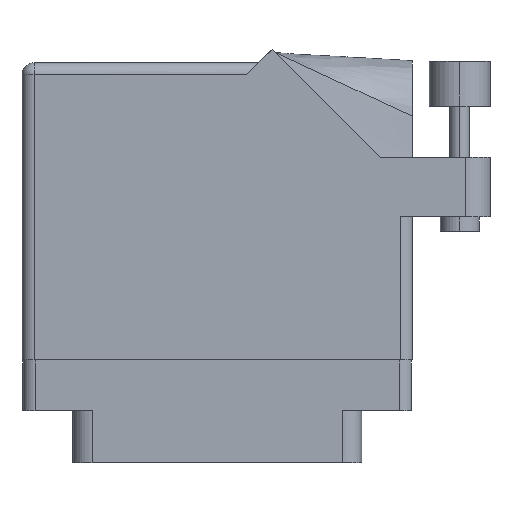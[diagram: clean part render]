
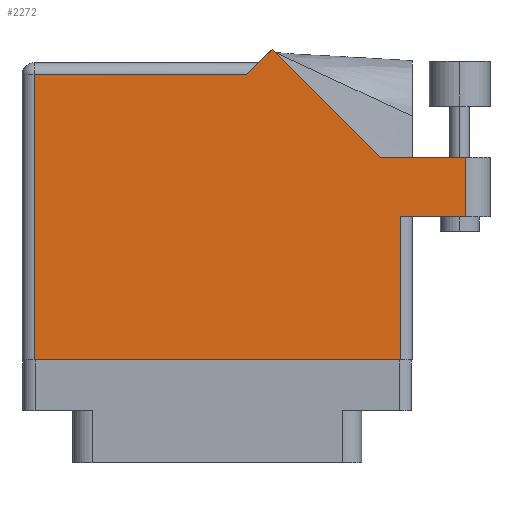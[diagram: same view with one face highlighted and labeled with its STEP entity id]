
A CAD part, front view. The second image highlights one B-rep face of the part: STEP entity #2272.
In plain terms, the highlighted face is planar.
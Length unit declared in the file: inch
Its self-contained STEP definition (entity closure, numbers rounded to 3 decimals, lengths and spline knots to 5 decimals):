
#702 = LINE ( 'NONE', #13015, #9710 ) ;
#1072 = DIRECTION ( 'NONE',  ( -0.707, 0.707, 0. ) ) ;
#1419 = CARTESIAN_POINT ( 'NONE',  ( 1.28771, 1.60071, 0. ) ) ;
#2039 = CARTESIAN_POINT ( 'NONE',  ( 1.948, 0.737, 0. ) ) ;
#2272 = ADVANCED_FACE ( 'NONE', ( #17366 ), #23611, .F. ) ;
#2548 = DIRECTION ( 'NONE',  ( 0., 0., -1. ) ) ;
#2586 = AXIS2_PLACEMENT_3D ( 'NONE', #30344, #2548, #4826 ) ;
#2947 = ORIENTED_EDGE ( 'NONE', *, *, #27175, .T. ) ;
#3048 = VECTOR ( 'NONE', #11093, 39.37008 ) ;
#3707 = CARTESIAN_POINT ( 'NONE',  ( 1.948, 0.737, 0. ) ) ;
#3743 = CARTESIAN_POINT ( 'NONE',  ( 2.285, 0.737, 0. ) ) ;
#4639 = DIRECTION ( 'NONE',  ( 1., 0., 0. ) ) ;
#4816 = CARTESIAN_POINT ( 'NONE',  ( 0.062, 1.468, 0. ) ) ;
#4826 = DIRECTION ( 'NONE',  ( -1., 0., 0. ) ) ;
#6056 = VERTEX_POINT ( 'NONE', #13619 ) ;
#6892 = DIRECTION ( 'NONE',  ( 1., 0., 0. ) ) ;
#6984 = VERTEX_POINT ( 'NONE', #25923 ) ;
#8253 = DIRECTION ( 'NONE',  ( -0.707, -0.707, 0. ) ) ;
#8354 = CARTESIAN_POINT ( 'NONE',  ( 1.84442, 1.044, 0. ) ) ;
#8413 = LINE ( 'NONE', #28722, #28688 ) ;
#9272 = VECTOR ( 'NONE', #6892, 39.37008 ) ;
#9411 = LINE ( 'NONE', #15979, #3048 ) ;
#9710 = VECTOR ( 'NONE', #1072, 39.37008 ) ;
#10117 = CARTESIAN_POINT ( 'NONE',  ( 2.285, 1.044, 0. ) ) ;
#10292 = VERTEX_POINT ( 'NONE', #4816 ) ;
#10432 = DIRECTION ( 'NONE',  ( 0., 1., 0. ) ) ;
#11093 = DIRECTION ( 'NONE',  ( 0., -1., 0. ) ) ;
#11745 = CARTESIAN_POINT ( 'NONE',  ( 2.01, 0.737, 0. ) ) ;
#12101 = ORIENTED_EDGE ( 'NONE', *, *, #15664, .T. ) ;
#13015 = CARTESIAN_POINT ( 'NONE',  ( 1.84442, 1.044, 0. ) ) ;
#13281 = CARTESIAN_POINT ( 'NONE',  ( 2.41, 1.044, 0. ) ) ;
#13391 = DIRECTION ( 'NONE',  ( -1., 0., 0. ) ) ;
#13619 = CARTESIAN_POINT ( 'NONE',  ( 0.062, 0., 0. ) ) ;
#13822 = VERTEX_POINT ( 'NONE', #1419 ) ;
#14353 = VECTOR ( 'NONE', #13391, 39.37008 ) ;
#15296 = VERTEX_POINT ( 'NONE', #20180 ) ;
#15664 = EDGE_CURVE ( 'NONE', #15296, #10292, #8413, .T. ) ;
#15979 = CARTESIAN_POINT ( 'NONE',  ( 0.062, 0., 0. ) ) ;
#16388 = LINE ( 'NONE', #2039, #27612 ) ;
#17276 = EDGE_CURVE ( 'NONE', #6984, #21477, #27123, .T. ) ;
#17366 = FACE_OUTER_BOUND ( 'NONE', #18644, .T. ) ;
#17962 = LINE ( 'NONE', #24942, #30354 ) ;
#18219 = VERTEX_POINT ( 'NONE', #3707 ) ;
#18430 = ORIENTED_EDGE ( 'NONE', *, *, #26678, .T. ) ;
#18644 = EDGE_LOOP ( 'NONE', ( #23502, #18430, #31048, #25879, #19253, #12101, #25400, #2947, #30390 ) ) ;
#19153 = EDGE_CURVE ( 'NONE', #10292, #6056, #9411, .T. ) ;
#19253 = ORIENTED_EDGE ( 'NONE', *, *, #28691, .T. ) ;
#19453 = CARTESIAN_POINT ( 'NONE',  ( 1.948, 0., 0. ) ) ;
#20180 = CARTESIAN_POINT ( 'NONE',  ( 1.155, 1.468, 0. ) ) ;
#21407 = DIRECTION ( 'NONE',  ( 0., 1., 0. ) ) ;
#21477 = VERTEX_POINT ( 'NONE', #8354 ) ;
#21483 = DIRECTION ( 'NONE',  ( -1., 0., 0. ) ) ;
#22442 = VECTOR ( 'NONE', #10432, 39.37008 ) ;
#23502 = ORIENTED_EDGE ( 'NONE', *, *, #24246, .T. ) ;
#23611 = PLANE ( 'NONE',  #2586 ) ;
#24246 = EDGE_CURVE ( 'NONE', #18219, #25685, #29378, .T. ) ;
#24713 = LINE ( 'NONE', #10117, #22442 ) ;
#24942 = CARTESIAN_POINT ( 'NONE',  ( 1.217, 1.53, 0. ) ) ;
#25400 = ORIENTED_EDGE ( 'NONE', *, *, #19153, .T. ) ;
#25685 = VERTEX_POINT ( 'NONE', #3743 ) ;
#25879 = ORIENTED_EDGE ( 'NONE', *, *, #26257, .T. ) ;
#25923 = CARTESIAN_POINT ( 'NONE',  ( 2.285, 1.044, 0. ) ) ;
#25981 = CARTESIAN_POINT ( 'NONE',  ( 0., 0., 0. ) ) ;
#26257 = EDGE_CURVE ( 'NONE', #21477, #13822, #702, .T. ) ;
#26678 = EDGE_CURVE ( 'NONE', #25685, #6984, #24713, .T. ) ;
#27123 = LINE ( 'NONE', #13281, #14353 ) ;
#27175 = EDGE_CURVE ( 'NONE', #6056, #29616, #28429, .T. ) ;
#27612 = VECTOR ( 'NONE', #21407, 39.37008 ) ;
#27784 = EDGE_CURVE ( 'NONE', #29616, #18219, #16388, .T. ) ;
#27885 = VECTOR ( 'NONE', #4639, 39.37008 ) ;
#28429 = LINE ( 'NONE', #25981, #9272 ) ;
#28688 = VECTOR ( 'NONE', #21483, 39.37008 ) ;
#28691 = EDGE_CURVE ( 'NONE', #13822, #15296, #17962, .T. ) ;
#28722 = CARTESIAN_POINT ( 'NONE',  ( 0., 1.468, 0. ) ) ;
#29378 = LINE ( 'NONE', #11745, #27885 ) ;
#29616 = VERTEX_POINT ( 'NONE', #19453 ) ;
#30344 = CARTESIAN_POINT ( 'NONE',  ( 0., 1.53, 0. ) ) ;
#30354 = VECTOR ( 'NONE', #8253, 39.37008 ) ;
#30390 = ORIENTED_EDGE ( 'NONE', *, *, #27784, .T. ) ;
#31048 = ORIENTED_EDGE ( 'NONE', *, *, #17276, .T. ) ;
